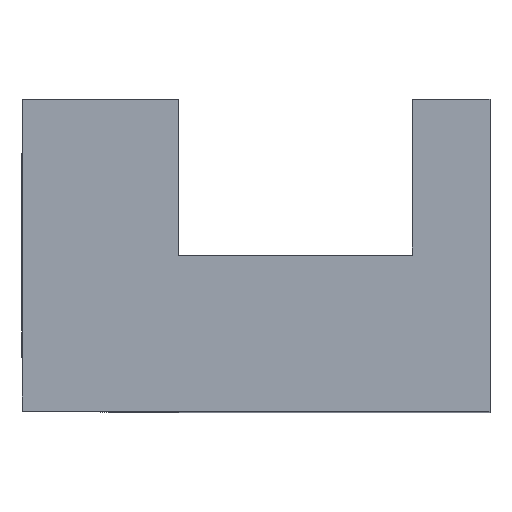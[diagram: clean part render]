
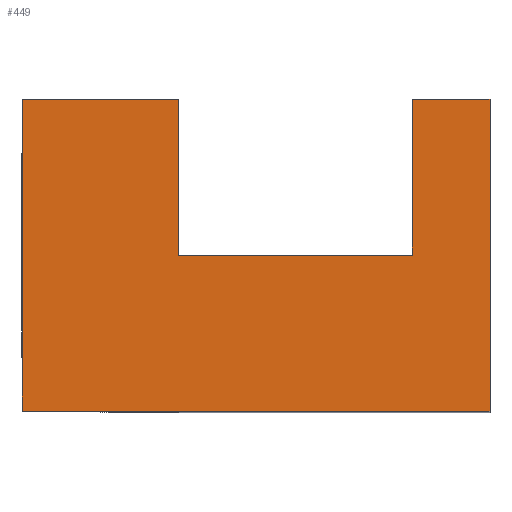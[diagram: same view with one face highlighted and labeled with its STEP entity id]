
A CAD part, top view. The second image highlights one B-rep face of the part: STEP entity #449.
In plain terms, the highlighted planar face has unit normal (0, 0, 1).
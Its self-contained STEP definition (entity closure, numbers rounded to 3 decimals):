
#2 = VERTEX_POINT ( 'NONE', #700 ) ;
#19 = ORIENTED_EDGE ( 'NONE', *, *, #387, .F. ) ;
#34 = VERTEX_POINT ( 'NONE', #711 ) ;
#77 = VERTEX_POINT ( 'NONE', #695 ) ;
#87 = DIRECTION ( 'NONE',  ( -1., 0., 0. ) ) ;
#108 = CARTESIAN_POINT ( 'NONE',  ( 26.754, 5.398, -3.546 ) ) ;
#138 = EDGE_CURVE ( 'NONE', #710, #598, #808, .T. ) ;
#140 = CARTESIAN_POINT ( 'NONE',  ( 26.754, 5.398, -3.546 ) ) ;
#175 = ORIENTED_EDGE ( 'NONE', *, *, #407, .F. ) ;
#179 = VERTEX_POINT ( 'NONE', #640 ) ;
#319 = VERTEX_POINT ( 'NONE', #140 ) ;
#325 = EDGE_CURVE ( 'NONE', #319, #34, #616, .T. ) ;
#377 = EDGE_CURVE ( 'NONE', #576, #710, #834, .T. ) ;
#387 = EDGE_CURVE ( 'NONE', #576, #2, #586, .T. ) ;
#389 = AXIS2_PLACEMENT_3D ( 'NONE', #618, #603, #601 ) ;
#394 = EDGE_CURVE ( 'NONE', #598, #77, #619, .T. ) ;
#407 = EDGE_CURVE ( 'NONE', #179, #77, #553, .T. ) ;
#411 = EDGE_CURVE ( 'NONE', #319, #179, #542, .T. ) ;
#413 = EDGE_CURVE ( 'NONE', #2, #34, #554, .T. ) ;
#449 = ADVANCED_FACE ( 'NONE', ( #511 ), #610, .F. ) ;
#480 = ORIENTED_EDGE ( 'NONE', *, *, #325, .T. ) ;
#488 = ORIENTED_EDGE ( 'NONE', *, *, #411, .F. ) ;
#497 = ORIENTED_EDGE ( 'NONE', *, *, #377, .T. ) ;
#504 = CARTESIAN_POINT ( 'NONE',  ( 11.754, 5.398, -3.546 ) ) ;
#511 = FACE_OUTER_BOUND ( 'NONE', #831, .T. ) ;
#523 = DIRECTION ( 'NONE',  ( -1., 0., 0. ) ) ;
#540 = VECTOR ( 'NONE', #666, 1000. ) ;
#542 = LINE ( 'NONE', #674, #548 ) ;
#548 = VECTOR ( 'NONE', #673, 1000. ) ;
#553 = LINE ( 'NONE', #691, #565 ) ;
#554 = LINE ( 'NONE', #692, #540 ) ;
#565 = VECTOR ( 'NONE', #690, 1000. ) ;
#567 = VECTOR ( 'NONE', #801, 1000. ) ;
#576 = VERTEX_POINT ( 'NONE', #583 ) ;
#579 = CARTESIAN_POINT ( 'NONE',  ( 4.254, 5.398, -3.546 ) ) ;
#583 = CARTESIAN_POINT ( 'NONE',  ( 11.754, -2.102, -3.546 ) ) ;
#586 = LINE ( 'NONE', #792, #567 ) ;
#594 = VECTOR ( 'NONE', #787, 1000. ) ;
#596 = VECTOR ( 'NONE', #799, 1000. ) ;
#598 = VERTEX_POINT ( 'NONE', #579 ) ;
#601 = DIRECTION ( 'NONE',  ( -1., 0., 0. ) ) ;
#602 = VECTOR ( 'NONE', #87, 1000. ) ;
#603 = DIRECTION ( 'NONE',  ( 0., 0., -1. ) ) ;
#610 = PLANE ( 'NONE',  #389 ) ;
#616 = LINE ( 'NONE', #108, #602 ) ;
#618 = CARTESIAN_POINT ( 'NONE',  ( 26.754, 5.398, -3.546 ) ) ;
#619 = LINE ( 'NONE', #791, #594 ) ;
#624 = ORIENTED_EDGE ( 'NONE', *, *, #394, .T. ) ;
#640 = CARTESIAN_POINT ( 'NONE',  ( 26.754, -9.602, -3.546 ) ) ;
#666 = DIRECTION ( 'NONE',  ( 0., 1., 0. ) ) ;
#668 = ORIENTED_EDGE ( 'NONE', *, *, #138, .T. ) ;
#671 = ORIENTED_EDGE ( 'NONE', *, *, #413, .F. ) ;
#673 = DIRECTION ( 'NONE',  ( 0., -1., 0. ) ) ;
#674 = CARTESIAN_POINT ( 'NONE',  ( 26.754, 5.398, -3.546 ) ) ;
#690 = DIRECTION ( 'NONE',  ( -1., 0., 0. ) ) ;
#691 = CARTESIAN_POINT ( 'NONE',  ( 26.754, -9.602, -3.546 ) ) ;
#692 = CARTESIAN_POINT ( 'NONE',  ( 23.004, -2.102, -3.546 ) ) ;
#695 = CARTESIAN_POINT ( 'NONE',  ( 4.254, -9.602, -3.546 ) ) ;
#700 = CARTESIAN_POINT ( 'NONE',  ( 23.004, -2.102, -3.546 ) ) ;
#706 = VECTOR ( 'NONE', #523, 1000. ) ;
#710 = VERTEX_POINT ( 'NONE', #504 ) ;
#711 = CARTESIAN_POINT ( 'NONE',  ( 23.004, 5.398, -3.546 ) ) ;
#720 = CARTESIAN_POINT ( 'NONE',  ( 26.754, 5.398, -3.546 ) ) ;
#787 = DIRECTION ( 'NONE',  ( 0., -1., 0. ) ) ;
#791 = CARTESIAN_POINT ( 'NONE',  ( 4.254, 5.398, -3.546 ) ) ;
#792 = CARTESIAN_POINT ( 'NONE',  ( 11.754, -2.102, -3.546 ) ) ;
#799 = DIRECTION ( 'NONE',  ( 0., 1., 0. ) ) ;
#800 = CARTESIAN_POINT ( 'NONE',  ( 11.754, -2.102, -3.546 ) ) ;
#801 = DIRECTION ( 'NONE',  ( 1., 0., 0. ) ) ;
#808 = LINE ( 'NONE', #720, #706 ) ;
#831 = EDGE_LOOP ( 'NONE', ( #19, #497, #668, #624, #175, #488, #480, #671 ) ) ;
#834 = LINE ( 'NONE', #800, #596 ) ;
